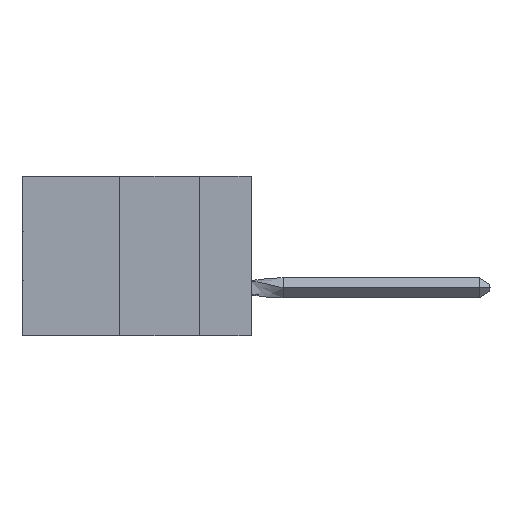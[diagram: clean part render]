
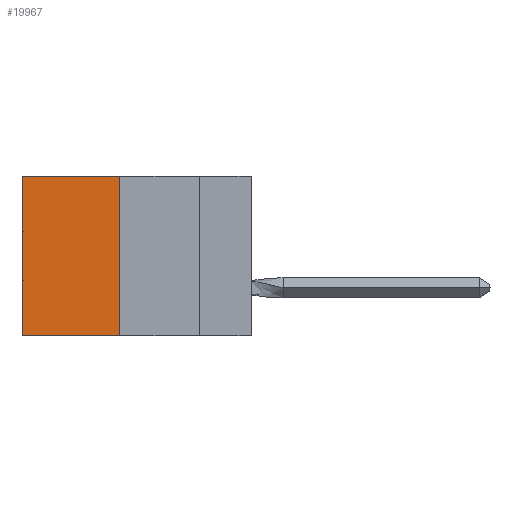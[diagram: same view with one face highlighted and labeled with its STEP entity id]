
A CAD part, left-side view. The second image highlights one B-rep face of the part: STEP entity #19967.
In plain terms, the highlighted planar face has unit normal (-1, 0, 0).
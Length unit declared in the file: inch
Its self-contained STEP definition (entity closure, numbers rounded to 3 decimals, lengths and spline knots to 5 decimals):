
#1758 = VECTOR ( 'NONE', #2896, 39.37008 ) ;
#2896 = DIRECTION ( 'NONE',  ( 0., 0., -1. ) ) ;
#3794 = CARTESIAN_POINT ( 'NONE',  ( 0.305, 0.72, 0. ) ) ;
#8927 = LINE ( 'NONE', #22392, #26522 ) ;
#9762 = CARTESIAN_POINT ( 'NONE',  ( 0.305, 0.413, 0. ) ) ;
#10179 = FACE_OUTER_BOUND ( 'NONE', #20342, .T. ) ;
#10854 = CARTESIAN_POINT ( 'NONE',  ( 0.305, 0.413, -0.5 ) ) ;
#11888 = VERTEX_POINT ( 'NONE', #10854 ) ;
#12333 = ORIENTED_EDGE ( 'NONE', *, *, #24789, .F. ) ;
#13405 = LINE ( 'NONE', #24927, #16549 ) ;
#15521 = CARTESIAN_POINT ( 'NONE',  ( 0.305, 0.413, -0.5 ) ) ;
#15628 = VERTEX_POINT ( 'NONE', #19377 ) ;
#16162 = LINE ( 'NONE', #9762, #23399 ) ;
#16549 = VECTOR ( 'NONE', #41595, 39.37008 ) ;
#17690 = AXIS2_PLACEMENT_3D ( 'NONE', #15521, #41596, #21750 ) ;
#17888 = EDGE_CURVE ( 'NONE', #11888, #30073, #13405, .T. ) ;
#19377 = CARTESIAN_POINT ( 'NONE',  ( 0.305, 0.413, 0. ) ) ;
#19967 = ADVANCED_FACE ( 'NONE', ( #10179 ), #25647, .F. ) ;
#20342 = EDGE_LOOP ( 'NONE', ( #24481, #33690, #12333, #30265 ) ) ;
#20611 = EDGE_CURVE ( 'NONE', #15628, #22775, #16162, .T. ) ;
#21750 = DIRECTION ( 'NONE',  ( 0., 0., -1. ) ) ;
#22392 = CARTESIAN_POINT ( 'NONE',  ( 0.305, 0.72, -0.5 ) ) ;
#22775 = VERTEX_POINT ( 'NONE', #3794 ) ;
#23106 = DIRECTION ( 'NONE',  ( 0., 1., 0. ) ) ;
#23399 = VECTOR ( 'NONE', #23106, 39.37008 ) ;
#24481 = ORIENTED_EDGE ( 'NONE', *, *, #27570, .T. ) ;
#24789 = EDGE_CURVE ( 'NONE', #15628, #11888, #31800, .T. ) ;
#24927 = CARTESIAN_POINT ( 'NONE',  ( 0.305, 0.413, -0.5 ) ) ;
#25647 = PLANE ( 'NONE',  #17690 ) ;
#26522 = VECTOR ( 'NONE', #41812, 39.37008 ) ;
#27570 = EDGE_CURVE ( 'NONE', #22775, #30073, #8927, .T. ) ;
#30073 = VERTEX_POINT ( 'NONE', #37808 ) ;
#30265 = ORIENTED_EDGE ( 'NONE', *, *, #20611, .T. ) ;
#31800 = LINE ( 'NONE', #38816, #1758 ) ;
#33690 = ORIENTED_EDGE ( 'NONE', *, *, #17888, .F. ) ;
#37808 = CARTESIAN_POINT ( 'NONE',  ( 0.305, 0.72, -0.5 ) ) ;
#38816 = CARTESIAN_POINT ( 'NONE',  ( 0.305, 0.413, -0.5 ) ) ;
#41595 = DIRECTION ( 'NONE',  ( 0., 1., 0. ) ) ;
#41596 = DIRECTION ( 'NONE',  ( 1., 0., 0. ) ) ;
#41812 = DIRECTION ( 'NONE',  ( 0., 0., -1. ) ) ;
